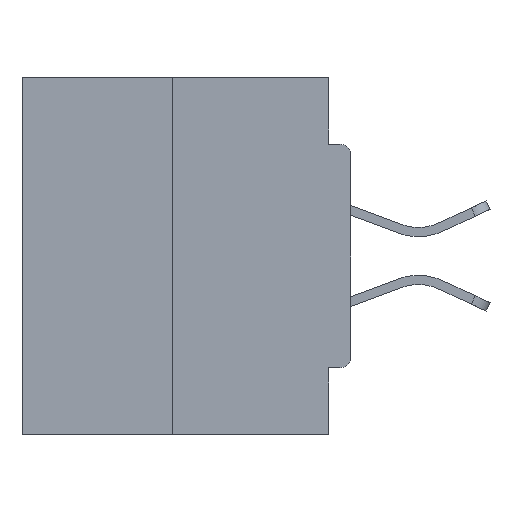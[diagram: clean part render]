
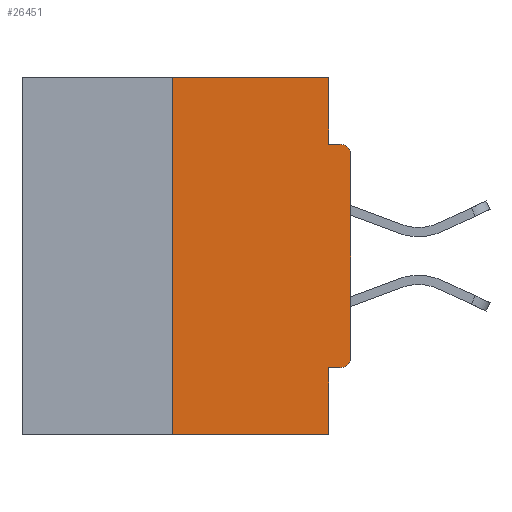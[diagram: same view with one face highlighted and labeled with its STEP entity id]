
A CAD part, left-side view. The second image highlights one B-rep face of the part: STEP entity #26451.
In plain terms, the highlighted planar face has unit normal (-1, 0, 0).
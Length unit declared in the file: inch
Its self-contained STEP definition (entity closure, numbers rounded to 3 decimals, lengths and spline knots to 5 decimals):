
#68 = EDGE_CURVE ( 'NONE', #5395, #19252, #23753, .T. ) ;
#239 = LINE ( 'NONE', #34001, #24662 ) ;
#1323 = CARTESIAN_POINT ( 'NONE',  ( 0., 0.46, -0.5 ) ) ;
#1684 = CARTESIAN_POINT ( 'NONE',  ( 0., 0., 0. ) ) ;
#1769 = DIRECTION ( 'NONE',  ( 0., -1., 0. ) ) ;
#1856 = ORIENTED_EDGE ( 'NONE', *, *, #25592, .F. ) ;
#2671 = CARTESIAN_POINT ( 'NONE',  ( 0., 0.031, -0.4065 ) ) ;
#3055 = CARTESIAN_POINT ( 'NONE',  ( 0., 0.031, -0.5 ) ) ;
#4102 = DIRECTION ( 'NONE',  ( 0., 0., -1. ) ) ;
#4878 = DIRECTION ( 'NONE',  ( 0., -1., 0. ) ) ;
#5395 = VERTEX_POINT ( 'NONE', #2671 ) ;
#6384 = CARTESIAN_POINT ( 'NONE',  ( 0., 0., -0.1085 ) ) ;
#6673 = ORIENTED_EDGE ( 'NONE', *, *, #29804, .T. ) ;
#6835 = CIRCLE ( 'NONE', #31846, 0.015 ) ;
#6850 = VERTEX_POINT ( 'NONE', #16167 ) ;
#8195 = DIRECTION ( 'NONE',  ( 0., 0., -1. ) ) ;
#8907 = EDGE_CURVE ( 'NONE', #34220, #24382, #27087, .T. ) ;
#10624 = CARTESIAN_POINT ( 'NONE',  ( 0., 0.015, -0.1085 ) ) ;
#11438 = CARTESIAN_POINT ( 'NONE',  ( 0., 0.015, -0.3915 ) ) ;
#11904 = CARTESIAN_POINT ( 'NONE',  ( 0., 0.031, 0. ) ) ;
#12187 = DIRECTION ( 'NONE',  ( 0., -1., 0. ) ) ;
#12281 = VERTEX_POINT ( 'NONE', #14077 ) ;
#12446 = EDGE_CURVE ( 'NONE', #6850, #33824, #17289, .T. ) ;
#12556 = PLANE ( 'NONE',  #26303 ) ;
#12636 = VERTEX_POINT ( 'NONE', #18670 ) ;
#12855 = CIRCLE ( 'NONE', #27015, 0.015 ) ;
#13355 = VECTOR ( 'NONE', #4878, 39.37008 ) ;
#13954 = FACE_OUTER_BOUND ( 'NONE', #23134, .T. ) ;
#14077 = CARTESIAN_POINT ( 'NONE',  ( 0., 0.015, -0.0935 ) ) ;
#14137 = VECTOR ( 'NONE', #1769, 39.37008 ) ;
#14344 = DIRECTION ( 'NONE',  ( -1., 0., 0. ) ) ;
#15289 = DIRECTION ( 'NONE',  ( 1., 0., 0. ) ) ;
#15451 = CARTESIAN_POINT ( 'NONE',  ( 0., 0.46, 0. ) ) ;
#15662 = ORIENTED_EDGE ( 'NONE', *, *, #20257, .F. ) ;
#16167 = CARTESIAN_POINT ( 'NONE',  ( 0., 0., -0.3915 ) ) ;
#17004 = ORIENTED_EDGE ( 'NONE', *, *, #12446, .T. ) ;
#17289 = LINE ( 'NONE', #1684, #22451 ) ;
#17602 = CARTESIAN_POINT ( 'NONE',  ( 0., 0.031, -0.5 ) ) ;
#17819 = DIRECTION ( 'NONE',  ( 0., 0., -1. ) ) ;
#18310 = VECTOR ( 'NONE', #33878, 39.37008 ) ;
#18670 = CARTESIAN_POINT ( 'NONE',  ( 0., 0.031, -0.0935 ) ) ;
#19149 = VERTEX_POINT ( 'NONE', #27827 ) ;
#19252 = VERTEX_POINT ( 'NONE', #17602 ) ;
#19953 = VERTEX_POINT ( 'NONE', #34685 ) ;
#20257 = EDGE_CURVE ( 'NONE', #24382, #12636, #34864, .T. ) ;
#20315 = VECTOR ( 'NONE', #8195, 39.37008 ) ;
#21070 = ORIENTED_EDGE ( 'NONE', *, *, #32226, .F. ) ;
#22213 = EDGE_CURVE ( 'NONE', #19149, #5395, #34274, .T. ) ;
#22233 = DIRECTION ( 'NONE',  ( 0., 0., -1. ) ) ;
#22451 = VECTOR ( 'NONE', #34413, 39.37008 ) ;
#22900 = EDGE_CURVE ( 'NONE', #33824, #12281, #6835, .T. ) ;
#23134 = EDGE_LOOP ( 'NONE', ( #23583, #21070, #6673, #32483, #27689, #24787, #17004, #30180, #1856, #15662 ) ) ;
#23149 = EDGE_CURVE ( 'NONE', #19149, #6850, #12855, .T. ) ;
#23583 = ORIENTED_EDGE ( 'NONE', *, *, #8907, .F. ) ;
#23753 = LINE ( 'NONE', #3055, #20315 ) ;
#24382 = VERTEX_POINT ( 'NONE', #26711 ) ;
#24550 = CARTESIAN_POINT ( 'NONE',  ( 0., 0., -0.4065 ) ) ;
#24662 = VECTOR ( 'NONE', #12187, 39.37008 ) ;
#24787 = ORIENTED_EDGE ( 'NONE', *, *, #23149, .T. ) ;
#25592 = EDGE_CURVE ( 'NONE', #12636, #12281, #239, .T. ) ;
#26303 = AXIS2_PLACEMENT_3D ( 'NONE', #31716, #15289, #17819 ) ;
#26451 = ADVANCED_FACE ( 'NONE', ( #13954 ), #12556, .F. ) ;
#26711 = CARTESIAN_POINT ( 'NONE',  ( 0., 0.031, 0. ) ) ;
#27015 = AXIS2_PLACEMENT_3D ( 'NONE', #11438, #14344, #22233 ) ;
#27087 = LINE ( 'NONE', #15451, #13355 ) ;
#27436 = DIRECTION ( 'NONE',  ( 0., 1., 0. ) ) ;
#27689 = ORIENTED_EDGE ( 'NONE', *, *, #22213, .F. ) ;
#27827 = CARTESIAN_POINT ( 'NONE',  ( 0., 0.015, -0.4065 ) ) ;
#27981 = CARTESIAN_POINT ( 'NONE',  ( 0., 0.25, 0. ) ) ;
#28241 = LINE ( 'NONE', #28758, #18310 ) ;
#28758 = CARTESIAN_POINT ( 'NONE',  ( 0., 0.25, 0. ) ) ;
#29804 = EDGE_CURVE ( 'NONE', #19953, #19252, #31685, .T. ) ;
#29834 = DIRECTION ( 'NONE',  ( -1., 0., 0. ) ) ;
#29948 = DIRECTION ( 'NONE',  ( 0., 0., -1. ) ) ;
#30180 = ORIENTED_EDGE ( 'NONE', *, *, #22900, .T. ) ;
#31685 = LINE ( 'NONE', #1323, #14137 ) ;
#31716 = CARTESIAN_POINT ( 'NONE',  ( 0., 0.46, 0. ) ) ;
#31846 = AXIS2_PLACEMENT_3D ( 'NONE', #10624, #29834, #29948 ) ;
#32226 = EDGE_CURVE ( 'NONE', #19953, #34220, #28241, .T. ) ;
#32483 = ORIENTED_EDGE ( 'NONE', *, *, #68, .F. ) ;
#33433 = VECTOR ( 'NONE', #27436, 39.37008 ) ;
#33609 = VECTOR ( 'NONE', #4102, 39.37008 ) ;
#33824 = VERTEX_POINT ( 'NONE', #6384 ) ;
#33878 = DIRECTION ( 'NONE',  ( 0., 0., 1. ) ) ;
#34001 = CARTESIAN_POINT ( 'NONE',  ( 0., 0., -0.0935 ) ) ;
#34220 = VERTEX_POINT ( 'NONE', #27981 ) ;
#34274 = LINE ( 'NONE', #24550, #33433 ) ;
#34413 = DIRECTION ( 'NONE',  ( 0., 0., 1. ) ) ;
#34685 = CARTESIAN_POINT ( 'NONE',  ( 0., 0.25, -0.5 ) ) ;
#34864 = LINE ( 'NONE', #11904, #33609 ) ;
